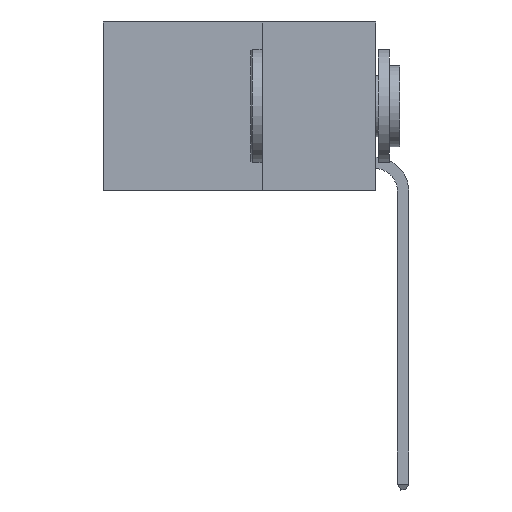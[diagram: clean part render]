
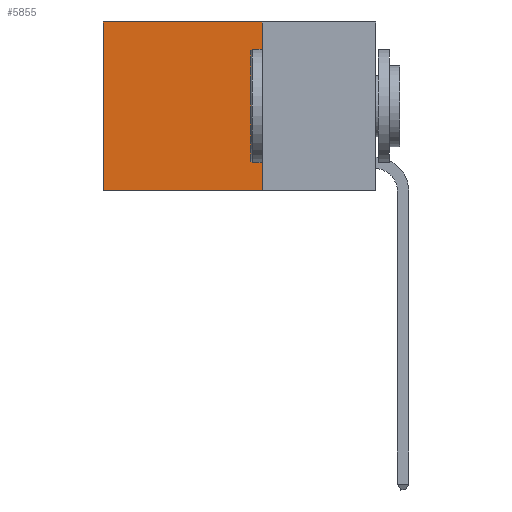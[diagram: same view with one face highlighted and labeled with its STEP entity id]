
A CAD part, left-side view. The second image highlights one B-rep face of the part: STEP entity #5855.
In plain terms, the highlighted planar face has unit normal (-1, 0, 0).
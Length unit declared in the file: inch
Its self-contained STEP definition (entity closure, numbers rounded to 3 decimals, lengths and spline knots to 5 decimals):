
#321 = DIRECTION ( 'NONE',  ( 1., 0., 0. ) ) ;
#1246 = CARTESIAN_POINT ( 'NONE',  ( 0.2625, 0.25, 0. ) ) ;
#1351 = ORIENTED_EDGE ( 'NONE', *, *, #7097, .T. ) ;
#2059 = LINE ( 'NONE', #6994, #12204 ) ;
#2187 = LINE ( 'NONE', #1246, #8974 ) ;
#2225 = FACE_OUTER_BOUND ( 'NONE', #7572, .T. ) ;
#2725 = CARTESIAN_POINT ( 'NONE',  ( 0.2625, 0.25, -0.37 ) ) ;
#3457 = CARTESIAN_POINT ( 'NONE',  ( 0.2625, 0.25, 0. ) ) ;
#3606 = EDGE_CURVE ( 'NONE', #6580, #5718, #2059, .T. ) ;
#3810 = DIRECTION ( 'NONE',  ( 0., 0., -1. ) ) ;
#3861 = DIRECTION ( 'NONE',  ( 0., 0., -1. ) ) ;
#4814 = LINE ( 'NONE', #4931, #7118 ) ;
#4931 = CARTESIAN_POINT ( 'NONE',  ( 0.2625, 0.25, 0. ) ) ;
#5012 = ORIENTED_EDGE ( 'NONE', *, *, #6617, .F. ) ;
#5718 = VERTEX_POINT ( 'NONE', #11546 ) ;
#5855 = ADVANCED_FACE ( 'NONE', ( #2225 ), #6163, .F. ) ;
#6150 = ORIENTED_EDGE ( 'NONE', *, *, #3606, .F. ) ;
#6163 = PLANE ( 'NONE',  #7919 ) ;
#6580 = VERTEX_POINT ( 'NONE', #2725 ) ;
#6617 = EDGE_CURVE ( 'NONE', #10271, #6580, #2187, .T. ) ;
#6908 = DIRECTION ( 'NONE',  ( 0., 0., -1. ) ) ;
#6994 = CARTESIAN_POINT ( 'NONE',  ( 0.2625, 0.25, -0.37 ) ) ;
#7097 = EDGE_CURVE ( 'NONE', #10271, #7532, #4814, .T. ) ;
#7118 = VECTOR ( 'NONE', #9961, 39.37008 ) ;
#7532 = VERTEX_POINT ( 'NONE', #8524 ) ;
#7572 = EDGE_LOOP ( 'NONE', ( #11654, #6150, #5012, #1351 ) ) ;
#7919 = AXIS2_PLACEMENT_3D ( 'NONE', #9118, #321, #6908 ) ;
#8524 = CARTESIAN_POINT ( 'NONE',  ( 0.2625, 0.6, 0. ) ) ;
#8712 = LINE ( 'NONE', #12602, #11263 ) ;
#8974 = VECTOR ( 'NONE', #3861, 39.37008 ) ;
#9118 = CARTESIAN_POINT ( 'NONE',  ( 0.2625, 0.25, 0. ) ) ;
#9911 = DIRECTION ( 'NONE',  ( 0., 1., 0. ) ) ;
#9961 = DIRECTION ( 'NONE',  ( 0., 1., 0. ) ) ;
#10271 = VERTEX_POINT ( 'NONE', #3457 ) ;
#10917 = EDGE_CURVE ( 'NONE', #7532, #5718, #8712, .T. ) ;
#11263 = VECTOR ( 'NONE', #3810, 39.37008 ) ;
#11546 = CARTESIAN_POINT ( 'NONE',  ( 0.2625, 0.6, -0.37 ) ) ;
#11654 = ORIENTED_EDGE ( 'NONE', *, *, #10917, .T. ) ;
#12204 = VECTOR ( 'NONE', #9911, 39.37008 ) ;
#12602 = CARTESIAN_POINT ( 'NONE',  ( 0.2625, 0.6, 0. ) ) ;
